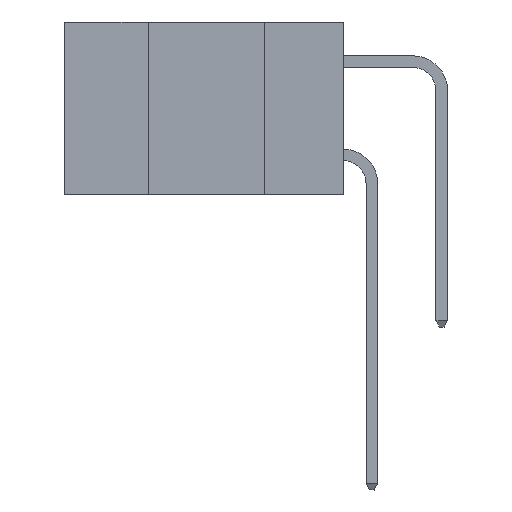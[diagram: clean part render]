
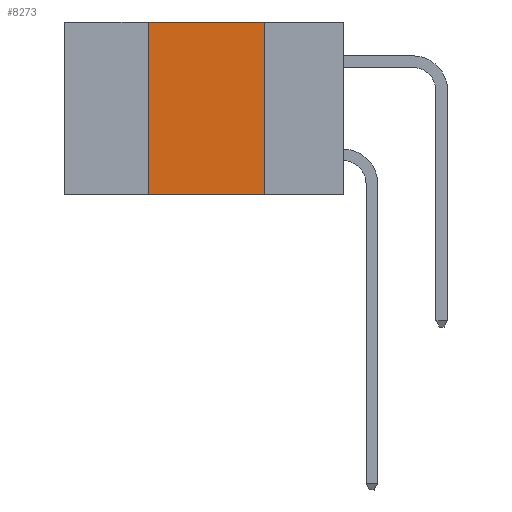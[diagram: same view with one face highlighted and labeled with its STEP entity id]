
A CAD part, left-side view. The second image highlights one B-rep face of the part: STEP entity #8273.
In plain terms, the highlighted planar face has unit normal (-1, 0, 0).
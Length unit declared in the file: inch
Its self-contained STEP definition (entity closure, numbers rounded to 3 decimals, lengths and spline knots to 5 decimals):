
#302 = ORIENTED_EDGE ( 'NONE', *, *, #15964, .F. ) ;
#522 = DIRECTION ( 'NONE',  ( 0., 0., 1. ) ) ;
#999 = VECTOR ( 'NONE', #9471, 39.37008 ) ;
#2021 = CARTESIAN_POINT ( 'NONE',  ( 0., 0.17, 0. ) ) ;
#2121 = DIRECTION ( 'NONE',  ( 1., 0., 0. ) ) ;
#2361 = CARTESIAN_POINT ( 'NONE',  ( 0., 0.17, 0. ) ) ;
#2658 = CARTESIAN_POINT ( 'NONE',  ( 0., 0.42, 0. ) ) ;
#2948 = LINE ( 'NONE', #2658, #9348 ) ;
#3926 = DIRECTION ( 'NONE',  ( 0., -1., 0. ) ) ;
#4058 = EDGE_LOOP ( 'NONE', ( #302, #5688, #22693, #17673 ) ) ;
#5688 = ORIENTED_EDGE ( 'NONE', *, *, #8824, .F. ) ;
#6775 = CARTESIAN_POINT ( 'NONE',  ( 0., 0.17, -0.37 ) ) ;
#7166 = VERTEX_POINT ( 'NONE', #17404 ) ;
#8273 = ADVANCED_FACE ( 'NONE', ( #17895 ), #16072, .F. ) ;
#8486 = CARTESIAN_POINT ( 'NONE',  ( 0., 0.6, 0. ) ) ;
#8824 = EDGE_CURVE ( 'NONE', #12566, #17057, #12742, .T. ) ;
#9348 = VECTOR ( 'NONE', #522, 39.37008 ) ;
#9471 = DIRECTION ( 'NONE',  ( 0., -1., 0. ) ) ;
#10177 = LINE ( 'NONE', #2021, #23397 ) ;
#10252 = CARTESIAN_POINT ( 'NONE',  ( 0., 0.42, 0. ) ) ;
#10616 = LINE ( 'NONE', #19650, #999 ) ;
#12299 = AXIS2_PLACEMENT_3D ( 'NONE', #8486, #2121, #18554 ) ;
#12566 = VERTEX_POINT ( 'NONE', #10252 ) ;
#12742 = LINE ( 'NONE', #16253, #14972 ) ;
#14143 = DIRECTION ( 'NONE',  ( 0., 0., -1. ) ) ;
#14972 = VECTOR ( 'NONE', #3926, 39.37008 ) ;
#15964 = EDGE_CURVE ( 'NONE', #17057, #26599, #10177, .T. ) ;
#16072 = PLANE ( 'NONE',  #12299 ) ;
#16253 = CARTESIAN_POINT ( 'NONE',  ( 0., 0.6, 0. ) ) ;
#17057 = VERTEX_POINT ( 'NONE', #2361 ) ;
#17404 = CARTESIAN_POINT ( 'NONE',  ( 0., 0.42, -0.37 ) ) ;
#17673 = ORIENTED_EDGE ( 'NONE', *, *, #18334, .T. ) ;
#17895 = FACE_OUTER_BOUND ( 'NONE', #4058, .T. ) ;
#18078 = EDGE_CURVE ( 'NONE', #7166, #12566, #2948, .T. ) ;
#18334 = EDGE_CURVE ( 'NONE', #7166, #26599, #10616, .T. ) ;
#18554 = DIRECTION ( 'NONE',  ( 0., 0., -1. ) ) ;
#19650 = CARTESIAN_POINT ( 'NONE',  ( 0., 0.6, -0.37 ) ) ;
#22693 = ORIENTED_EDGE ( 'NONE', *, *, #18078, .F. ) ;
#23397 = VECTOR ( 'NONE', #14143, 39.37008 ) ;
#26599 = VERTEX_POINT ( 'NONE', #6775 ) ;
